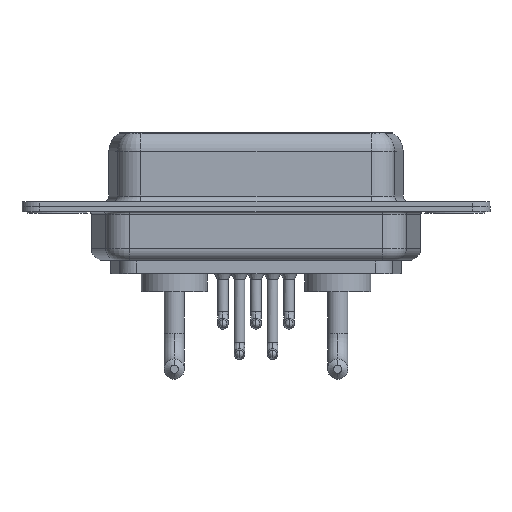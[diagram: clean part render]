
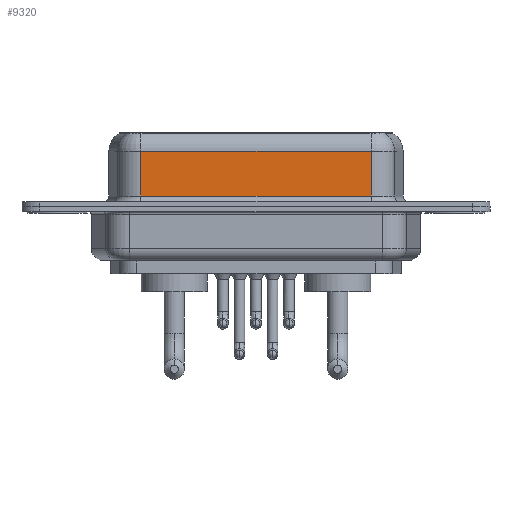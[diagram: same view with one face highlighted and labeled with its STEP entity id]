
A CAD part, front view. The second image highlights one B-rep face of the part: STEP entity #9320.
In plain terms, the highlighted planar face has unit normal (0, -1, 0).
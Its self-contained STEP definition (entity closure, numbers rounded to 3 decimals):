
#38 = CARTESIAN_POINT ( 'NONE',  ( 26.287, -3.95, 6.4 ) ) ;
#332 = CARTESIAN_POINT ( 'NONE',  ( 26.287, -3.95, 4.65 ) ) ;
#552 = VERTEX_POINT ( 'NONE', #332 ) ;
#755 = LINE ( 'NONE', #4204, #8603 ) ;
#1177 = FACE_OUTER_BOUND ( 'NONE', #10048, .T. ) ;
#1629 = DIRECTION ( 'NONE',  ( -1., 0., 0. ) ) ;
#1803 = CARTESIAN_POINT ( 'NONE',  ( 26.287, -3.95, 0.9 ) ) ;
#2246 = EDGE_CURVE ( 'NONE', #552, #15080, #8580, .T. ) ;
#2660 = ORIENTED_EDGE ( 'NONE', *, *, #2246, .T. ) ;
#2772 = EDGE_CURVE ( 'NONE', #552, #4174, #755, .T. ) ;
#2793 = ORIENTED_EDGE ( 'NONE', *, *, #12822, .T. ) ;
#2961 = CARTESIAN_POINT ( 'NONE',  ( 7.013, -3.95, 6.4 ) ) ;
#3916 = VECTOR ( 'NONE', #5166, 1000. ) ;
#4174 = VERTEX_POINT ( 'NONE', #7573 ) ;
#4204 = CARTESIAN_POINT ( 'NONE',  ( 26.287, -3.95, 6.4 ) ) ;
#4673 = VECTOR ( 'NONE', #1629, 1000. ) ;
#4778 = DIRECTION ( 'NONE',  ( 0., 1., 0. ) ) ;
#4891 = EDGE_CURVE ( 'NONE', #15080, #6891, #14491, .T. ) ;
#5166 = DIRECTION ( 'NONE',  ( 1., 0., 0. ) ) ;
#5249 = DIRECTION ( 'NONE',  ( 0., 0., -1. ) ) ;
#5843 = PLANE ( 'NONE',  #7537 ) ;
#6060 = CARTESIAN_POINT ( 'NONE',  ( 26.287, -3.95, 4.65 ) ) ;
#6511 = CARTESIAN_POINT ( 'NONE',  ( 7.013, -3.95, 0.9 ) ) ;
#6891 = VERTEX_POINT ( 'NONE', #6511 ) ;
#7537 = AXIS2_PLACEMENT_3D ( 'NONE', #38, #4778, #11506 ) ;
#7573 = CARTESIAN_POINT ( 'NONE',  ( 26.287, -3.95, 0.9 ) ) ;
#8580 = LINE ( 'NONE', #6060, #4673 ) ;
#8602 = LINE ( 'NONE', #1803, #3916 ) ;
#8603 = VECTOR ( 'NONE', #13287, 1000. ) ;
#9320 = ADVANCED_FACE ( 'NONE', ( #1177 ), #5843, .F. ) ;
#10048 = EDGE_LOOP ( 'NONE', ( #12449, #2660, #13744, #2793 ) ) ;
#11506 = DIRECTION ( 'NONE',  ( 0., 0., 1. ) ) ;
#11803 = CARTESIAN_POINT ( 'NONE',  ( 7.013, -3.95, 4.65 ) ) ;
#12449 = ORIENTED_EDGE ( 'NONE', *, *, #2772, .F. ) ;
#12822 = EDGE_CURVE ( 'NONE', #6891, #4174, #8602, .T. ) ;
#13287 = DIRECTION ( 'NONE',  ( 0., 0., -1. ) ) ;
#13744 = ORIENTED_EDGE ( 'NONE', *, *, #4891, .T. ) ;
#14491 = LINE ( 'NONE', #2961, #15006 ) ;
#15006 = VECTOR ( 'NONE', #5249, 1000. ) ;
#15080 = VERTEX_POINT ( 'NONE', #11803 ) ;
